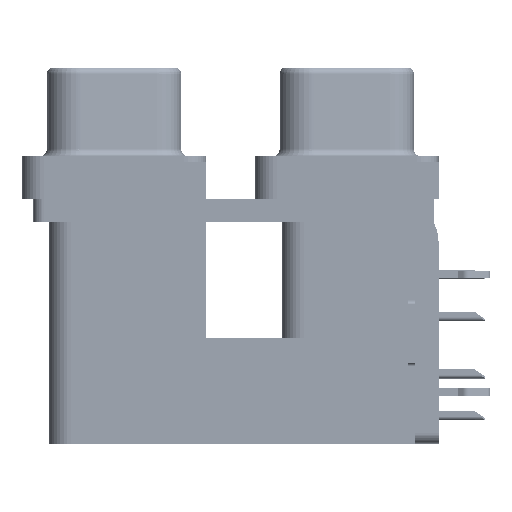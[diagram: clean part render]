
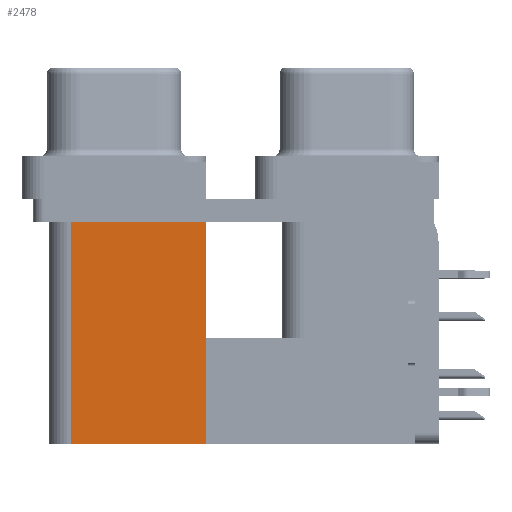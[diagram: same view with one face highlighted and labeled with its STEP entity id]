
A CAD part, left-side view. The second image highlights one B-rep face of the part: STEP entity #2478.
In plain terms, the highlighted planar face has unit normal (-1, 0, 0).
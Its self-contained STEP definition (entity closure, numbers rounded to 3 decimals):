
#913 = DIRECTION ( 'NONE',  ( 1., 0., 0. ) ) ;
#2478 = ADVANCED_FACE ( 'NONE', ( #21208 ), #46064, .F. ) ;
#3068 = VECTOR ( 'NONE', #26758, 1000. ) ;
#4173 = DIRECTION ( 'NONE',  ( 0., 0., 1. ) ) ;
#4203 = ORIENTED_EDGE ( 'NONE', *, *, #25814, .F. ) ;
#8882 = VECTOR ( 'NONE', #4173, 1000. ) ;
#9378 = ORIENTED_EDGE ( 'NONE', *, *, #23618, .T. ) ;
#17130 = CARTESIAN_POINT ( 'NONE',  ( 3.79, 9.6, -2.5 ) ) ;
#21208 = FACE_OUTER_BOUND ( 'NONE', #46947, .T. ) ;
#21525 = CARTESIAN_POINT ( 'NONE',  ( 3.79, 18.8, -19.2 ) ) ;
#23618 = EDGE_CURVE ( 'NONE', #24444, #47337, #44335, .T. ) ;
#24444 = VERTEX_POINT ( 'NONE', #17130 ) ;
#25081 = EDGE_CURVE ( 'NONE', #25227, #47337, #41031, .T. ) ;
#25227 = VERTEX_POINT ( 'NONE', #21525 ) ;
#25814 = EDGE_CURVE ( 'NONE', #50296, #25227, #30920, .T. ) ;
#26758 = DIRECTION ( 'NONE',  ( 0., 1., 0. ) ) ;
#30920 = LINE ( 'NONE', #52272, #42001 ) ;
#31727 = DIRECTION ( 'NONE',  ( 0., 1., 0. ) ) ;
#32021 = LINE ( 'NONE', #52557, #8882 ) ;
#35681 = CARTESIAN_POINT ( 'NONE',  ( 3.79, 9.6, -2.5 ) ) ;
#35907 = VECTOR ( 'NONE', #41292, 1000. ) ;
#41031 = LINE ( 'NONE', #44544, #35907 ) ;
#41292 = DIRECTION ( 'NONE',  ( 0., 0., 1. ) ) ;
#42001 = VECTOR ( 'NONE', #31727, 1000. ) ;
#42806 = AXIS2_PLACEMENT_3D ( 'NONE', #50414, #913, #45797 ) ;
#43278 = EDGE_CURVE ( 'NONE', #50296, #24444, #32021, .T. ) ;
#44335 = LINE ( 'NONE', #35681, #3068 ) ;
#44544 = CARTESIAN_POINT ( 'NONE',  ( 3.79, 18.8, -19.2 ) ) ;
#44681 = ORIENTED_EDGE ( 'NONE', *, *, #25081, .F. ) ;
#45797 = DIRECTION ( 'NONE',  ( 0., 0., -1. ) ) ;
#46064 = PLANE ( 'NONE',  #42806 ) ;
#46947 = EDGE_LOOP ( 'NONE', ( #9378, #44681, #4203, #50857 ) ) ;
#47337 = VERTEX_POINT ( 'NONE', #49683 ) ;
#49155 = CARTESIAN_POINT ( 'NONE',  ( 3.79, 9.6, -19.2 ) ) ;
#49683 = CARTESIAN_POINT ( 'NONE',  ( 3.79, 18.8, -2.5 ) ) ;
#50296 = VERTEX_POINT ( 'NONE', #49155 ) ;
#50414 = CARTESIAN_POINT ( 'NONE',  ( 3.79, 9.6, -19.2 ) ) ;
#50857 = ORIENTED_EDGE ( 'NONE', *, *, #43278, .T. ) ;
#52272 = CARTESIAN_POINT ( 'NONE',  ( 3.79, 9.6, -19.2 ) ) ;
#52557 = CARTESIAN_POINT ( 'NONE',  ( 3.79, 9.6, -19.2 ) ) ;
